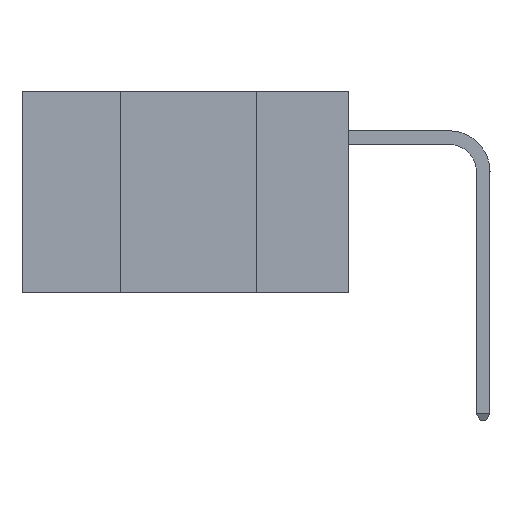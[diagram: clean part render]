
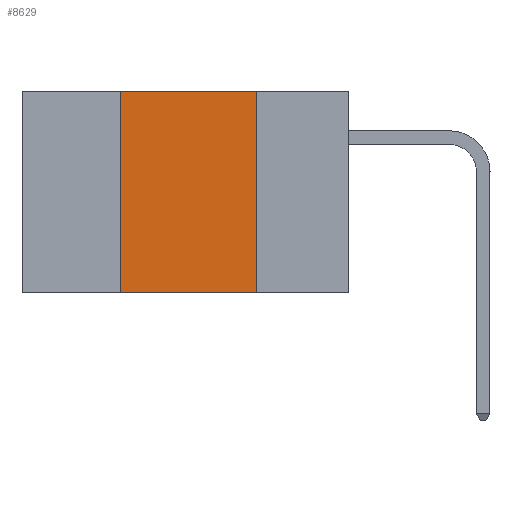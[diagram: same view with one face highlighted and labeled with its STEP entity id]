
A CAD part, left-side view. The second image highlights one B-rep face of the part: STEP entity #8629.
In plain terms, the highlighted planar face has unit normal (-1, 0, 0).
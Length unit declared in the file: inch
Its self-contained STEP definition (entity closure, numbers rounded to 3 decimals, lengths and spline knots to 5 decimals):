
#637 = LINE ( 'NONE', #15015, #3547 ) ;
#1922 = VERTEX_POINT ( 'NONE', #2847 ) ;
#2097 = EDGE_CURVE ( 'NONE', #12805, #12121, #5659, .T. ) ;
#2446 = LINE ( 'NONE', #17090, #12886 ) ;
#2762 = DIRECTION ( 'NONE',  ( 0., 0., -1. ) ) ;
#2842 = FACE_OUTER_BOUND ( 'NONE', #5685, .T. ) ;
#2847 = CARTESIAN_POINT ( 'NONE',  ( 0., 0.17, 0. ) ) ;
#3547 = VECTOR ( 'NONE', #15108, 39.37008 ) ;
#3704 = EDGE_CURVE ( 'NONE', #12805, #16390, #637, .T. ) ;
#3726 = ORIENTED_EDGE ( 'NONE', *, *, #2097, .T. ) ;
#5318 = LINE ( 'NONE', #13176, #12502 ) ;
#5659 = LINE ( 'NONE', #12635, #8645 ) ;
#5685 = EDGE_LOOP ( 'NONE', ( #15289, #7340, #7889, #3726 ) ) ;
#7242 = CARTESIAN_POINT ( 'NONE',  ( 0., 0.42, 0. ) ) ;
#7340 = ORIENTED_EDGE ( 'NONE', *, *, #8469, .F. ) ;
#7889 = ORIENTED_EDGE ( 'NONE', *, *, #3704, .F. ) ;
#8469 = EDGE_CURVE ( 'NONE', #16390, #1922, #5318, .T. ) ;
#8629 = ADVANCED_FACE ( 'NONE', ( #2842 ), #10862, .F. ) ;
#8645 = VECTOR ( 'NONE', #9887, 39.37008 ) ;
#9887 = DIRECTION ( 'NONE',  ( 0., -1., 0. ) ) ;
#10029 = CARTESIAN_POINT ( 'NONE',  ( 0., 0.17, -0.37 ) ) ;
#10862 = PLANE ( 'NONE',  #11395 ) ;
#11395 = AXIS2_PLACEMENT_3D ( 'NONE', #13588, #14839, #2762 ) ;
#11928 = DIRECTION ( 'NONE',  ( 0., -1., 0. ) ) ;
#12121 = VERTEX_POINT ( 'NONE', #10029 ) ;
#12502 = VECTOR ( 'NONE', #11928, 39.37008 ) ;
#12635 = CARTESIAN_POINT ( 'NONE',  ( 0., 0.6, -0.37 ) ) ;
#12805 = VERTEX_POINT ( 'NONE', #16435 ) ;
#12886 = VECTOR ( 'NONE', #16841, 39.37008 ) ;
#13176 = CARTESIAN_POINT ( 'NONE',  ( 0., 0.6, 0. ) ) ;
#13588 = CARTESIAN_POINT ( 'NONE',  ( 0., 0.6, 0. ) ) ;
#13769 = EDGE_CURVE ( 'NONE', #1922, #12121, #2446, .T. ) ;
#14839 = DIRECTION ( 'NONE',  ( 1., 0., 0. ) ) ;
#15015 = CARTESIAN_POINT ( 'NONE',  ( 0., 0.42, 0. ) ) ;
#15108 = DIRECTION ( 'NONE',  ( 0., 0., 1. ) ) ;
#15289 = ORIENTED_EDGE ( 'NONE', *, *, #13769, .F. ) ;
#16390 = VERTEX_POINT ( 'NONE', #7242 ) ;
#16435 = CARTESIAN_POINT ( 'NONE',  ( 0., 0.42, -0.37 ) ) ;
#16841 = DIRECTION ( 'NONE',  ( 0., 0., -1. ) ) ;
#17090 = CARTESIAN_POINT ( 'NONE',  ( 0., 0.17, 0. ) ) ;
